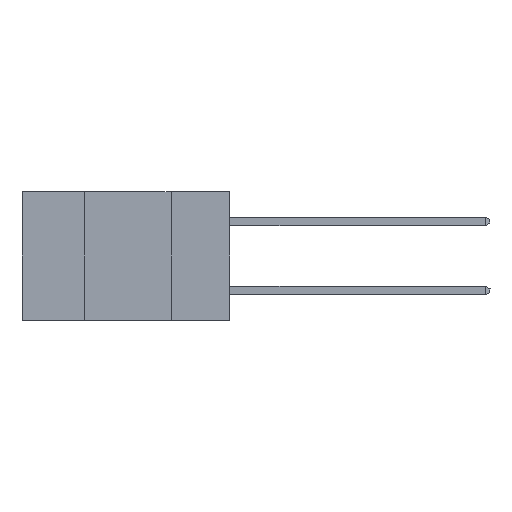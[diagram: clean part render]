
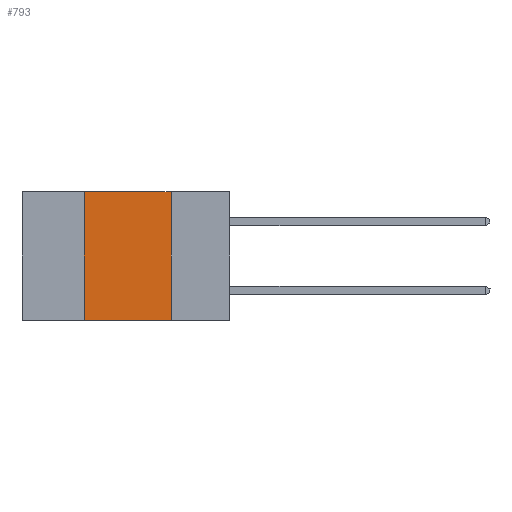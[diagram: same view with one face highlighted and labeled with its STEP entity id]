
A CAD part, left-side view. The second image highlights one B-rep face of the part: STEP entity #793.
In plain terms, the highlighted planar face has unit normal (-1, 0, 0).
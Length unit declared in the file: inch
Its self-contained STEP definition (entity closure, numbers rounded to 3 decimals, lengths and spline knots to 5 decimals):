
#374 = VECTOR ( 'NONE', #18113, 39.37008 ) ;
#793 = ADVANCED_FACE ( 'NONE', ( #5090 ), #16559, .F. ) ;
#1245 = EDGE_CURVE ( 'NONE', #10427, #11128, #15528, .T. ) ;
#2242 = ORIENTED_EDGE ( 'NONE', *, *, #7382, .T. ) ;
#2765 = ORIENTED_EDGE ( 'NONE', *, *, #1245, .F. ) ;
#2948 = AXIS2_PLACEMENT_3D ( 'NONE', #5694, #3612, #12201 ) ;
#3561 = CARTESIAN_POINT ( 'NONE',  ( 0., 0.6, -0.37 ) ) ;
#3612 = DIRECTION ( 'NONE',  ( 1., 0., 0. ) ) ;
#3860 = LINE ( 'NONE', #3561, #20116 ) ;
#4722 = VECTOR ( 'NONE', #19943, 39.37008 ) ;
#5090 = FACE_OUTER_BOUND ( 'NONE', #8656, .T. ) ;
#5694 = CARTESIAN_POINT ( 'NONE',  ( 0., 0.6, 0. ) ) ;
#5861 = CARTESIAN_POINT ( 'NONE',  ( 0., 0.17, -0.37 ) ) ;
#7270 = CARTESIAN_POINT ( 'NONE',  ( 0., 0.42, 0. ) ) ;
#7382 = EDGE_CURVE ( 'NONE', #25838, #11128, #3860, .T. ) ;
#8656 = EDGE_LOOP ( 'NONE', ( #2765, #23390, #14630, #2242 ) ) ;
#8709 = CARTESIAN_POINT ( 'NONE',  ( 0., 0.42, -0.37 ) ) ;
#9384 = EDGE_CURVE ( 'NONE', #25838, #11708, #15277, .T. ) ;
#10084 = DIRECTION ( 'NONE',  ( 0., -1., 0. ) ) ;
#10427 = VERTEX_POINT ( 'NONE', #26337 ) ;
#11128 = VERTEX_POINT ( 'NONE', #5861 ) ;
#11708 = VERTEX_POINT ( 'NONE', #7270 ) ;
#12201 = DIRECTION ( 'NONE',  ( 0., 0., -1. ) ) ;
#14630 = ORIENTED_EDGE ( 'NONE', *, *, #9384, .F. ) ;
#15277 = LINE ( 'NONE', #15926, #374 ) ;
#15528 = LINE ( 'NONE', #20313, #4722 ) ;
#15618 = EDGE_CURVE ( 'NONE', #11708, #10427, #26772, .T. ) ;
#15926 = CARTESIAN_POINT ( 'NONE',  ( 0., 0.42, 0. ) ) ;
#16147 = CARTESIAN_POINT ( 'NONE',  ( 0., 0.6, 0. ) ) ;
#16559 = PLANE ( 'NONE',  #2948 ) ;
#18113 = DIRECTION ( 'NONE',  ( 0., 0., 1. ) ) ;
#19943 = DIRECTION ( 'NONE',  ( 0., 0., -1. ) ) ;
#20116 = VECTOR ( 'NONE', #10084, 39.37008 ) ;
#20313 = CARTESIAN_POINT ( 'NONE',  ( 0., 0.17, 0. ) ) ;
#20326 = VECTOR ( 'NONE', #21147, 39.37008 ) ;
#21147 = DIRECTION ( 'NONE',  ( 0., -1., 0. ) ) ;
#23390 = ORIENTED_EDGE ( 'NONE', *, *, #15618, .F. ) ;
#25838 = VERTEX_POINT ( 'NONE', #8709 ) ;
#26337 = CARTESIAN_POINT ( 'NONE',  ( 0., 0.17, 0. ) ) ;
#26772 = LINE ( 'NONE', #16147, #20326 ) ;
